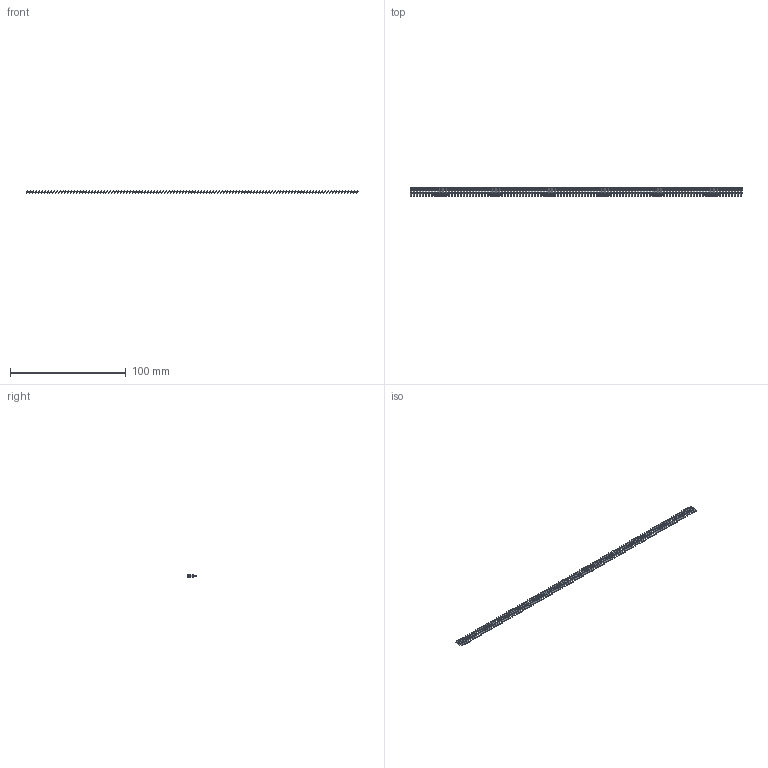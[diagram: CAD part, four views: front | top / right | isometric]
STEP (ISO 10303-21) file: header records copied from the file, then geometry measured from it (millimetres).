
FILE_DESCRIPTION (( 'STEP AP203' ), '1' );
FILE_NAME ('106-113-253-100.STEP', '2020-04-16T23:38:14', ( '' ), ( '' ), 'SwSTEP 2.0', 'SolidWorks 2016', '' );
FILE_SCHEMA (( 'CONFIG_CONTROL_DESIGN' ));
Length unit declared in the file: inch
Products named in the file (2): 106-113-253-100; 100-290-001_100-290-253
Assembly tree (113 placements, depth 2):
  106-113-253-100
    100-290-001_100-290-253  x113
Bounding box: 286.28 x 7.62 x 1.8 mm (x, y, z)
Volume: 623.5 mm3; surface area: 3888 mm2
Topology: 113 solids, 113 shells, 2260 faces, 6102 edges, 4068 vertices
Faces by surface type: plane 2147, cylinder 113
Entity records: 4404 total; most frequent: DIRECTION 328, CALENDAR_DATE 236, DATE_AND_TIME 236, COORDINATED_UNIVERSAL_TIME_OFFSET 236, LOCAL_TIME 236, CARTESIAN_POINT 226, AXIS2_PLACEMENT_3D 138, PERSON_AND_ORGANIZATION 129
